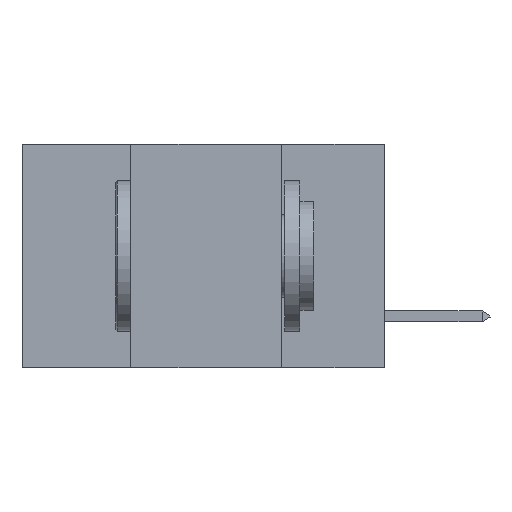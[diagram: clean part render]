
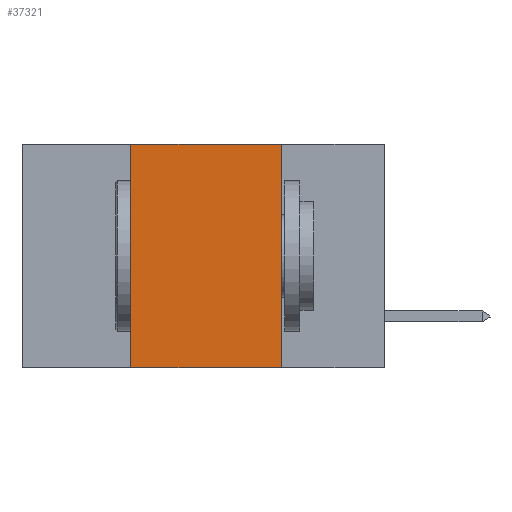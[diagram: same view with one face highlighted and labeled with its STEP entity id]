
A CAD part, left-side view. The second image highlights one B-rep face of the part: STEP entity #37321.
In plain terms, the highlighted planar face has unit normal (-1, 0, 0).
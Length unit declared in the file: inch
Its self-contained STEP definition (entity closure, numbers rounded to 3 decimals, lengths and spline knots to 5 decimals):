
#891 = ORIENTED_EDGE ( 'NONE', *, *, #6461, .T. ) ;
#3136 = VECTOR ( 'NONE', #43092, 39.37008 ) ;
#4418 = EDGE_CURVE ( 'NONE', #19635, #14581, #10199, .T. ) ;
#4684 = EDGE_CURVE ( 'NONE', #14581, #14008, #26226, .T. ) ;
#5792 = CARTESIAN_POINT ( 'NONE',  ( 0., 0.6, -0.37 ) ) ;
#6461 = EDGE_CURVE ( 'NONE', #19635, #11838, #19211, .T. ) ;
#7275 = CARTESIAN_POINT ( 'NONE',  ( 0., 0.6, 0. ) ) ;
#9530 = VECTOR ( 'NONE', #14277, 39.37008 ) ;
#9566 = DIRECTION ( 'NONE',  ( 1., 0., 0. ) ) ;
#10199 = LINE ( 'NONE', #29327, #23590 ) ;
#10782 = CARTESIAN_POINT ( 'NONE',  ( 0., 0.42, 0. ) ) ;
#11838 = VERTEX_POINT ( 'NONE', #12761 ) ;
#12759 = DIRECTION ( 'NONE',  ( 0., 0., -1. ) ) ;
#12761 = CARTESIAN_POINT ( 'NONE',  ( 0., 0.17, -0.37 ) ) ;
#14008 = VERTEX_POINT ( 'NONE', #33297 ) ;
#14277 = DIRECTION ( 'NONE',  ( 0., 0., -1. ) ) ;
#14581 = VERTEX_POINT ( 'NONE', #10782 ) ;
#18052 = EDGE_CURVE ( 'NONE', #14008, #11838, #42113, .T. ) ;
#19211 = LINE ( 'NONE', #5792, #3136 ) ;
#19635 = VERTEX_POINT ( 'NONE', #31009 ) ;
#20386 = VECTOR ( 'NONE', #33245, 39.37008 ) ;
#22832 = ORIENTED_EDGE ( 'NONE', *, *, #18052, .F. ) ;
#23590 = VECTOR ( 'NONE', #43195, 39.37008 ) ;
#26226 = LINE ( 'NONE', #7275, #20386 ) ;
#28260 = CARTESIAN_POINT ( 'NONE',  ( 0., 0.17, 0. ) ) ;
#29327 = CARTESIAN_POINT ( 'NONE',  ( 0., 0.42, 0. ) ) ;
#31009 = CARTESIAN_POINT ( 'NONE',  ( 0., 0.42, -0.37 ) ) ;
#31670 = AXIS2_PLACEMENT_3D ( 'NONE', #39882, #9566, #12759 ) ;
#32856 = PLANE ( 'NONE',  #31670 ) ;
#33070 = ORIENTED_EDGE ( 'NONE', *, *, #4418, .F. ) ;
#33245 = DIRECTION ( 'NONE',  ( 0., -1., 0. ) ) ;
#33297 = CARTESIAN_POINT ( 'NONE',  ( 0., 0.17, 0. ) ) ;
#35383 = ORIENTED_EDGE ( 'NONE', *, *, #4684, .F. ) ;
#37321 = ADVANCED_FACE ( 'NONE', ( #41917 ), #32856, .F. ) ;
#39882 = CARTESIAN_POINT ( 'NONE',  ( 0., 0.6, 0. ) ) ;
#40718 = EDGE_LOOP ( 'NONE', ( #22832, #35383, #33070, #891 ) ) ;
#41917 = FACE_OUTER_BOUND ( 'NONE', #40718, .T. ) ;
#42113 = LINE ( 'NONE', #28260, #9530 ) ;
#43092 = DIRECTION ( 'NONE',  ( 0., -1., 0. ) ) ;
#43195 = DIRECTION ( 'NONE',  ( 0., 0., 1. ) ) ;
